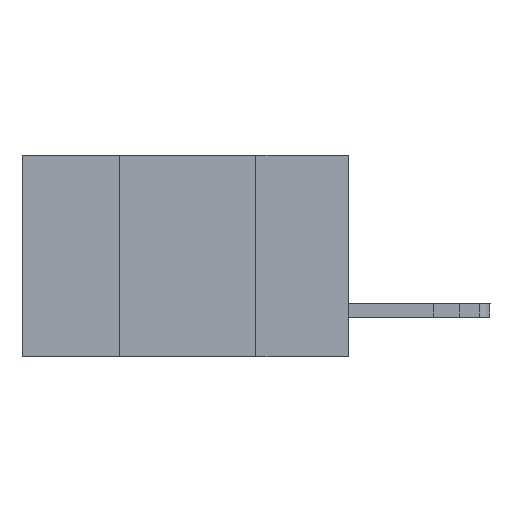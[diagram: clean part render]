
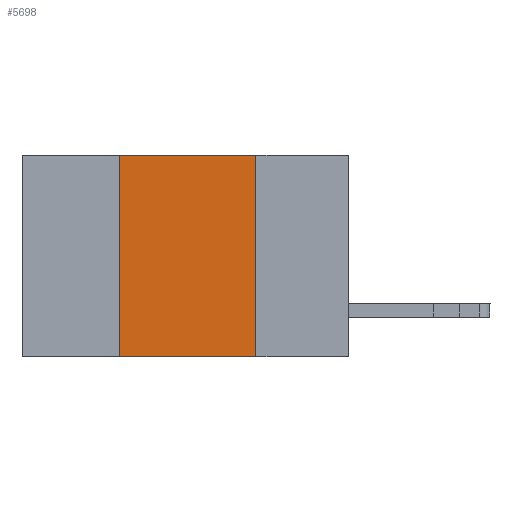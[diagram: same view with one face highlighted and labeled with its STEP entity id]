
A CAD part, left-side view. The second image highlights one B-rep face of the part: STEP entity #5698.
In plain terms, the highlighted planar face has unit normal (-1, 0, 0).
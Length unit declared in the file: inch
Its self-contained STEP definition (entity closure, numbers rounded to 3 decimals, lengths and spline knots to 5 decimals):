
#152 = VECTOR ( 'NONE', #2073, 39.37008 ) ;
#475 = CARTESIAN_POINT ( 'NONE',  ( 0., 0.17, -0.37 ) ) ;
#817 = CARTESIAN_POINT ( 'NONE',  ( 0., 0.6, 0. ) ) ;
#869 = PLANE ( 'NONE',  #11224 ) ;
#1094 = CARTESIAN_POINT ( 'NONE',  ( 0., 0.6, 0. ) ) ;
#1273 = CARTESIAN_POINT ( 'NONE',  ( 0., 0.42, 0. ) ) ;
#1512 = DIRECTION ( 'NONE',  ( 0., 0., 1. ) ) ;
#1683 = EDGE_CURVE ( 'NONE', #11108, #7452, #11453, .T. ) ;
#2073 = DIRECTION ( 'NONE',  ( 0., -1., 0. ) ) ;
#2484 = CARTESIAN_POINT ( 'NONE',  ( 0., 0.42, -0.37 ) ) ;
#2535 = EDGE_CURVE ( 'NONE', #11108, #4772, #4262, .T. ) ;
#3801 = CARTESIAN_POINT ( 'NONE',  ( 0., 0.17, -0.37 ) ) ;
#4027 = DIRECTION ( 'NONE',  ( 0., 0., -1. ) ) ;
#4229 = VECTOR ( 'NONE', #1512, 39.37008 ) ;
#4262 = LINE ( 'NONE', #4365, #6937 ) ;
#4365 = CARTESIAN_POINT ( 'NONE',  ( 0., 0.6, -0.37 ) ) ;
#4430 = EDGE_CURVE ( 'NONE', #7452, #11280, #10754, .T. ) ;
#4772 = VERTEX_POINT ( 'NONE', #3801 ) ;
#4940 = ORIENTED_EDGE ( 'NONE', *, *, #6518, .F. ) ;
#5269 = DIRECTION ( 'NONE',  ( 1., 0., 0. ) ) ;
#5698 = ADVANCED_FACE ( 'NONE', ( #6871 ), #869, .F. ) ;
#6104 = DIRECTION ( 'NONE',  ( 0., 0., -1. ) ) ;
#6518 = EDGE_CURVE ( 'NONE', #11280, #4772, #8453, .T. ) ;
#6871 = FACE_OUTER_BOUND ( 'NONE', #9561, .T. ) ;
#6937 = VECTOR ( 'NONE', #9736, 39.37008 ) ;
#7031 = ORIENTED_EDGE ( 'NONE', *, *, #2535, .T. ) ;
#7452 = VERTEX_POINT ( 'NONE', #1273 ) ;
#8117 = VECTOR ( 'NONE', #4027, 39.37008 ) ;
#8453 = LINE ( 'NONE', #475, #8117 ) ;
#9265 = ORIENTED_EDGE ( 'NONE', *, *, #4430, .F. ) ;
#9561 = EDGE_LOOP ( 'NONE', ( #4940, #9265, #10269, #7031 ) ) ;
#9736 = DIRECTION ( 'NONE',  ( 0., -1., 0. ) ) ;
#10269 = ORIENTED_EDGE ( 'NONE', *, *, #1683, .F. ) ;
#10677 = CARTESIAN_POINT ( 'NONE',  ( 0., 0.42, -0.37 ) ) ;
#10754 = LINE ( 'NONE', #1094, #152 ) ;
#11019 = CARTESIAN_POINT ( 'NONE',  ( 0., 0.17, 0. ) ) ;
#11108 = VERTEX_POINT ( 'NONE', #10677 ) ;
#11224 = AXIS2_PLACEMENT_3D ( 'NONE', #817, #5269, #6104 ) ;
#11280 = VERTEX_POINT ( 'NONE', #11019 ) ;
#11453 = LINE ( 'NONE', #2484, #4229 ) ;
